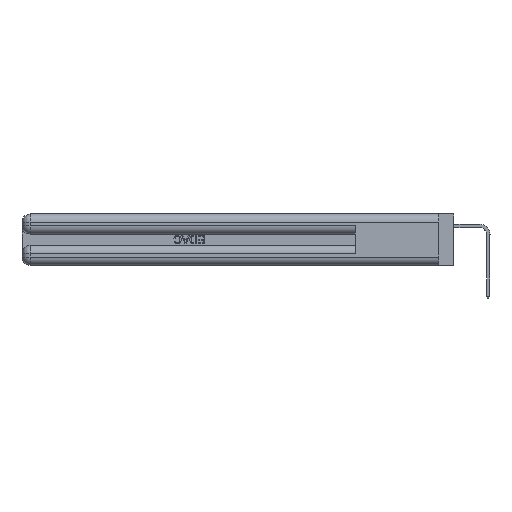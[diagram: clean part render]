
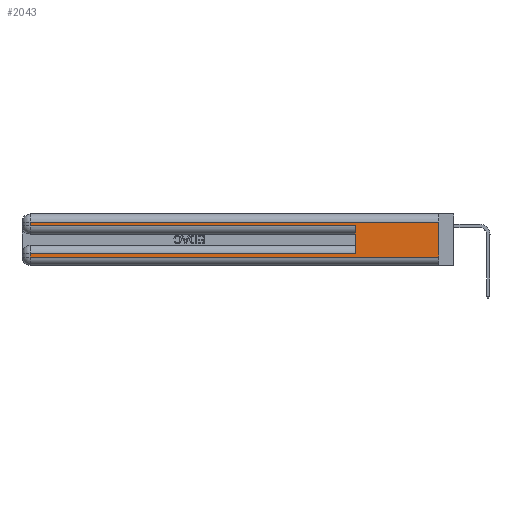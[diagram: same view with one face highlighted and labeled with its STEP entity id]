
A CAD part, left-side view. The second image highlights one B-rep face of the part: STEP entity #2043.
In plain terms, the highlighted planar face has unit normal (-1, 0, 0).
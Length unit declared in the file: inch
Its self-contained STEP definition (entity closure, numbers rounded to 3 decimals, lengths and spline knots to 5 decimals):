
#320 = ORIENTED_EDGE ( 'NONE', *, *, #32720, .F. ) ;
#645 = EDGE_CURVE ( 'NONE', #25932, #18716, #18404, .T. ) ;
#753 = VERTEX_POINT ( 'NONE', #3643 ) ;
#921 = EDGE_CURVE ( 'NONE', #33736, #28692, #33477, .T. ) ;
#1515 = CARTESIAN_POINT ( 'NONE',  ( 0., 0.6, 0.145 ) ) ;
#2043 = ADVANCED_FACE ( 'NONE', ( #40585 ), #33128, .F. ) ;
#2203 = ORIENTED_EDGE ( 'NONE', *, *, #22773, .F. ) ;
#2433 = VECTOR ( 'NONE', #35505, 39.37008 ) ;
#3643 = CARTESIAN_POINT ( 'NONE',  ( 0., 2.94, 0.06 ) ) ;
#4402 = LINE ( 'NONE', #33712, #41302 ) ;
#5148 = DIRECTION ( 'NONE',  ( 0., 0., 1. ) ) ;
#5807 = VECTOR ( 'NONE', #25586, 39.37008 ) ;
#6661 = DIRECTION ( 'NONE',  ( 0., 0., -1. ) ) ;
#6737 = VERTEX_POINT ( 'NONE', #11395 ) ;
#6920 = CARTESIAN_POINT ( 'NONE',  ( 0., 0., 0.285 ) ) ;
#10255 = CARTESIAN_POINT ( 'NONE',  ( 0., 2.94, 0.37 ) ) ;
#10506 = CARTESIAN_POINT ( 'NONE',  ( 0., 0., 0.31 ) ) ;
#10520 = DIRECTION ( 'NONE',  ( 0., -1., 0. ) ) ;
#10715 = CARTESIAN_POINT ( 'NONE',  ( 0., 0., 0.06 ) ) ;
#10736 = VECTOR ( 'NONE', #10520, 39.37008 ) ;
#11395 = CARTESIAN_POINT ( 'NONE',  ( 0., 0., 0.06 ) ) ;
#12170 = ORIENTED_EDGE ( 'NONE', *, *, #645, .T. ) ;
#12408 = EDGE_CURVE ( 'NONE', #28692, #753, #43810, .T. ) ;
#14014 = ORIENTED_EDGE ( 'NONE', *, *, #12408, .T. ) ;
#14245 = ORIENTED_EDGE ( 'NONE', *, *, #29026, .T. ) ;
#14437 = VECTOR ( 'NONE', #22473, 39.37008 ) ;
#14462 = VECTOR ( 'NONE', #39289, 39.37008 ) ;
#15292 = DIRECTION ( 'NONE',  ( 0., 0., -1. ) ) ;
#16120 = CARTESIAN_POINT ( 'NONE',  ( 0., 0., 0.31 ) ) ;
#16623 = VECTOR ( 'NONE', #5148, 39.37008 ) ;
#18404 = LINE ( 'NONE', #10255, #44619 ) ;
#18716 = VERTEX_POINT ( 'NONE', #31465 ) ;
#18747 = CARTESIAN_POINT ( 'NONE',  ( 0., 0., 0.37 ) ) ;
#18849 = CARTESIAN_POINT ( 'NONE',  ( 0., 0., 0.085 ) ) ;
#19088 = CARTESIAN_POINT ( 'NONE',  ( 0., 0.6, 0.085 ) ) ;
#20902 = ORIENTED_EDGE ( 'NONE', *, *, #32923, .T. ) ;
#21529 = LINE ( 'NONE', #10506, #2433 ) ;
#22026 = CARTESIAN_POINT ( 'NONE',  ( 0., 2.94, 0.085 ) ) ;
#22473 = DIRECTION ( 'NONE',  ( 0., 1., 0. ) ) ;
#22773 = EDGE_CURVE ( 'NONE', #33736, #36310, #45088, .T. ) ;
#25120 = LINE ( 'NONE', #10715, #14462 ) ;
#25586 = DIRECTION ( 'NONE',  ( 0., 0., -1. ) ) ;
#25932 = VERTEX_POINT ( 'NONE', #45283 ) ;
#27159 = ORIENTED_EDGE ( 'NONE', *, *, #921, .T. ) ;
#28692 = VERTEX_POINT ( 'NONE', #22026 ) ;
#29026 = EDGE_CURVE ( 'NONE', #35859, #25932, #21529, .T. ) ;
#29647 = AXIS2_PLACEMENT_3D ( 'NONE', #18747, #36699, #15292 ) ;
#31465 = CARTESIAN_POINT ( 'NONE',  ( 0., 2.94, 0.285 ) ) ;
#32506 = CARTESIAN_POINT ( 'NONE',  ( 0., 0.6, 0.285 ) ) ;
#32720 = EDGE_CURVE ( 'NONE', #35859, #6737, #4402, .T. ) ;
#32923 = EDGE_CURVE ( 'NONE', #753, #6737, #25120, .T. ) ;
#33128 = PLANE ( 'NONE',  #29647 ) ;
#33477 = LINE ( 'NONE', #18849, #14437 ) ;
#33634 = ORIENTED_EDGE ( 'NONE', *, *, #37307, .T. ) ;
#33712 = CARTESIAN_POINT ( 'NONE',  ( 0., 0., 0.37 ) ) ;
#33736 = VERTEX_POINT ( 'NONE', #19088 ) ;
#35505 = DIRECTION ( 'NONE',  ( 0., 1., 0. ) ) ;
#35859 = VERTEX_POINT ( 'NONE', #16120 ) ;
#36310 = VERTEX_POINT ( 'NONE', #32506 ) ;
#36699 = DIRECTION ( 'NONE',  ( 1., 0., 0. ) ) ;
#37307 = EDGE_CURVE ( 'NONE', #18716, #36310, #39231, .T. ) ;
#39231 = LINE ( 'NONE', #6920, #10736 ) ;
#39289 = DIRECTION ( 'NONE',  ( 0., -1., 0. ) ) ;
#40585 = FACE_OUTER_BOUND ( 'NONE', #42712, .T. ) ;
#41302 = VECTOR ( 'NONE', #44434, 39.37008 ) ;
#42712 = EDGE_LOOP ( 'NONE', ( #320, #14245, #12170, #33634, #2203, #27159, #14014, #20902 ) ) ;
#43330 = CARTESIAN_POINT ( 'NONE',  ( 0., 2.94, 0.37 ) ) ;
#43810 = LINE ( 'NONE', #43330, #5807 ) ;
#44434 = DIRECTION ( 'NONE',  ( 0., 0., -1. ) ) ;
#44619 = VECTOR ( 'NONE', #6661, 39.37008 ) ;
#45088 = LINE ( 'NONE', #1515, #16623 ) ;
#45283 = CARTESIAN_POINT ( 'NONE',  ( 0., 2.94, 0.31 ) ) ;
